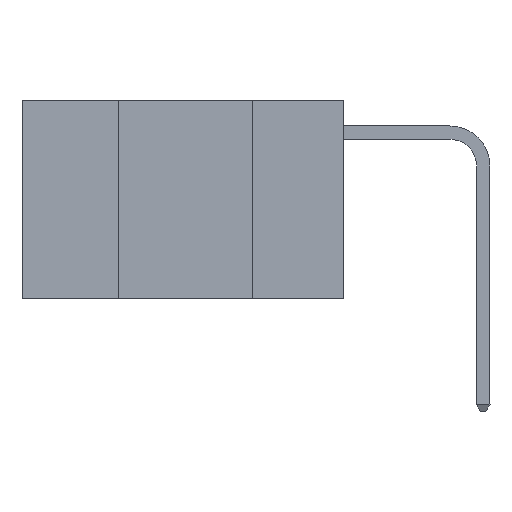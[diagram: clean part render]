
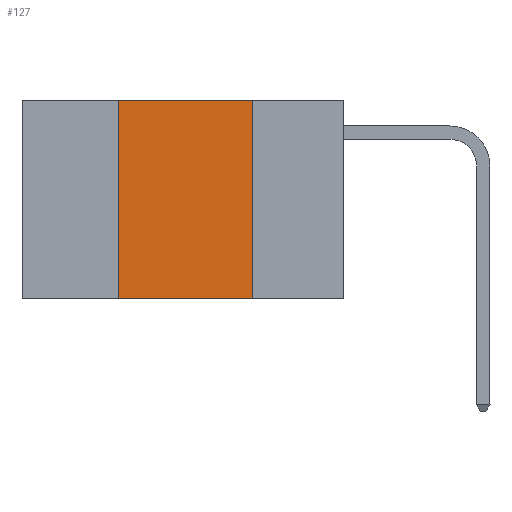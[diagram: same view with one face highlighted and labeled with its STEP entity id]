
A CAD part, left-side view. The second image highlights one B-rep face of the part: STEP entity #127.
In plain terms, the highlighted planar face has unit normal (-1, 0, 0).
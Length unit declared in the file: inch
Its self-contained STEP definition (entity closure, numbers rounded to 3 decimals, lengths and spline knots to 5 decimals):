
#14 = LINE ( 'NONE', #1816, #4380 ) ;
#127 = ADVANCED_FACE ( 'NONE', ( #9070 ), #4807, .F. ) ;
#622 = LINE ( 'NONE', #9113, #4996 ) ;
#641 = CARTESIAN_POINT ( 'NONE',  ( 0., 0.17, 0. ) ) ;
#814 = VERTEX_POINT ( 'NONE', #2009 ) ;
#951 = AXIS2_PLACEMENT_3D ( 'NONE', #3826, #1227, #7226 ) ;
#1011 = EDGE_LOOP ( 'NONE', ( #10297, #7884, #1535, #6814 ) ) ;
#1227 = DIRECTION ( 'NONE',  ( 1., 0., 0. ) ) ;
#1444 = EDGE_CURVE ( 'NONE', #6748, #814, #2418, .T. ) ;
#1535 = ORIENTED_EDGE ( 'NONE', *, *, #2314, .F. ) ;
#1656 = LINE ( 'NONE', #3497, #3005 ) ;
#1816 = CARTESIAN_POINT ( 'NONE',  ( 0., 0.6, -0.37 ) ) ;
#2009 = CARTESIAN_POINT ( 'NONE',  ( 0., 0.17, -0.37 ) ) ;
#2314 = EDGE_CURVE ( 'NONE', #10673, #4538, #1656, .T. ) ;
#2418 = LINE ( 'NONE', #7555, #6882 ) ;
#2529 = DIRECTION ( 'NONE',  ( 0., 0., -1. ) ) ;
#3005 = VECTOR ( 'NONE', #6833, 39.37008 ) ;
#3363 = DIRECTION ( 'NONE',  ( 0., -1., 0. ) ) ;
#3497 = CARTESIAN_POINT ( 'NONE',  ( 0., 0.42, 0. ) ) ;
#3826 = CARTESIAN_POINT ( 'NONE',  ( 0., 0.6, 0. ) ) ;
#3844 = EDGE_CURVE ( 'NONE', #4538, #6748, #622, .T. ) ;
#3985 = DIRECTION ( 'NONE',  ( 0., -1., 0. ) ) ;
#4380 = VECTOR ( 'NONE', #3363, 39.37008 ) ;
#4501 = CARTESIAN_POINT ( 'NONE',  ( 0., 0.42, 0. ) ) ;
#4538 = VERTEX_POINT ( 'NONE', #4501 ) ;
#4807 = PLANE ( 'NONE',  #951 ) ;
#4996 = VECTOR ( 'NONE', #3985, 39.37008 ) ;
#6748 = VERTEX_POINT ( 'NONE', #641 ) ;
#6814 = ORIENTED_EDGE ( 'NONE', *, *, #9967, .T. ) ;
#6833 = DIRECTION ( 'NONE',  ( 0., 0., 1. ) ) ;
#6882 = VECTOR ( 'NONE', #2529, 39.37008 ) ;
#7226 = DIRECTION ( 'NONE',  ( 0., 0., -1. ) ) ;
#7555 = CARTESIAN_POINT ( 'NONE',  ( 0., 0.17, 0. ) ) ;
#7884 = ORIENTED_EDGE ( 'NONE', *, *, #3844, .F. ) ;
#8984 = CARTESIAN_POINT ( 'NONE',  ( 0., 0.42, -0.37 ) ) ;
#9070 = FACE_OUTER_BOUND ( 'NONE', #1011, .T. ) ;
#9113 = CARTESIAN_POINT ( 'NONE',  ( 0., 0.6, 0. ) ) ;
#9967 = EDGE_CURVE ( 'NONE', #10673, #814, #14, .T. ) ;
#10297 = ORIENTED_EDGE ( 'NONE', *, *, #1444, .F. ) ;
#10673 = VERTEX_POINT ( 'NONE', #8984 ) ;
